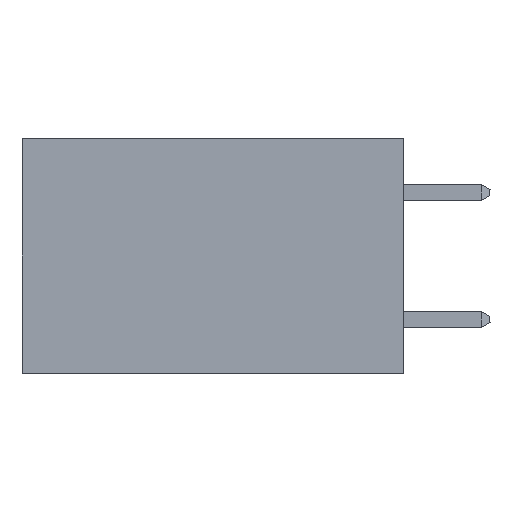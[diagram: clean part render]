
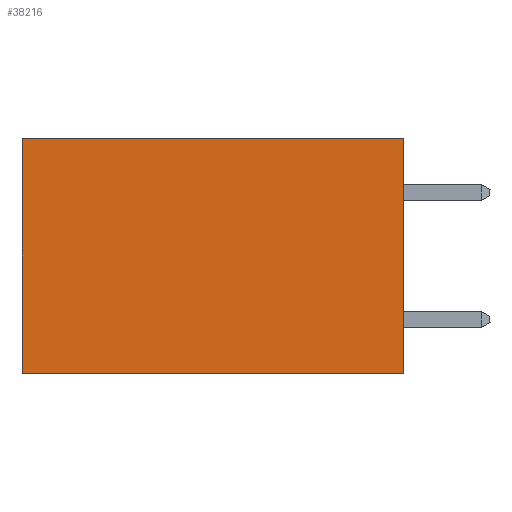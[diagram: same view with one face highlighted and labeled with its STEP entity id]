
A CAD part, left-side view. The second image highlights one B-rep face of the part: STEP entity #38216.
In plain terms, the highlighted planar face has unit normal (-1, 0, 0).
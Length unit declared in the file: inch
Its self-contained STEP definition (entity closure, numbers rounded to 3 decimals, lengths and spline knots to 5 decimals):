
#215 = CARTESIAN_POINT ( 'NONE',  ( 0.2875, 0., 0. ) ) ;
#1062 = DIRECTION ( 'NONE',  ( 0., 0., -1. ) ) ;
#1606 = EDGE_LOOP ( 'NONE', ( #6245, #32530, #17756, #23178 ) ) ;
#1956 = CARTESIAN_POINT ( 'NONE',  ( 0.2875, 0.6, -0.37 ) ) ;
#2699 = EDGE_CURVE ( 'NONE', #33863, #4896, #27996, .T. ) ;
#3627 = CARTESIAN_POINT ( 'NONE',  ( 0.2875, 0., -0.37 ) ) ;
#4805 = VECTOR ( 'NONE', #36527, 39.37008 ) ;
#4896 = VERTEX_POINT ( 'NONE', #1956 ) ;
#5256 = LINE ( 'NONE', #39238, #4805 ) ;
#6245 = ORIENTED_EDGE ( 'NONE', *, *, #2699, .T. ) ;
#9655 = VERTEX_POINT ( 'NONE', #215 ) ;
#12582 = CARTESIAN_POINT ( 'NONE',  ( 0.2875, 0., 0. ) ) ;
#15834 = PLANE ( 'NONE',  #16896 ) ;
#16367 = VECTOR ( 'NONE', #32789, 39.37008 ) ;
#16896 = AXIS2_PLACEMENT_3D ( 'NONE', #12582, #28119, #18883 ) ;
#17756 = ORIENTED_EDGE ( 'NONE', *, *, #39743, .F. ) ;
#18292 = FACE_OUTER_BOUND ( 'NONE', #1606, .T. ) ;
#18370 = VECTOR ( 'NONE', #1062, 39.37008 ) ;
#18883 = DIRECTION ( 'NONE',  ( 0., 0., -1. ) ) ;
#20125 = CARTESIAN_POINT ( 'NONE',  ( 0.2875, 0.6, 0. ) ) ;
#20802 = VECTOR ( 'NONE', #36061, 39.37008 ) ;
#23178 = ORIENTED_EDGE ( 'NONE', *, *, #31960, .T. ) ;
#27996 = LINE ( 'NONE', #20125, #16367 ) ;
#28119 = DIRECTION ( 'NONE',  ( 1., 0., 0. ) ) ;
#30313 = CARTESIAN_POINT ( 'NONE',  ( 0.2875, 0., -0.37 ) ) ;
#30358 = VERTEX_POINT ( 'NONE', #3627 ) ;
#31385 = LINE ( 'NONE', #35011, #18370 ) ;
#31960 = EDGE_CURVE ( 'NONE', #9655, #33863, #5256, .T. ) ;
#32530 = ORIENTED_EDGE ( 'NONE', *, *, #39800, .F. ) ;
#32789 = DIRECTION ( 'NONE',  ( 0., 0., -1. ) ) ;
#33784 = LINE ( 'NONE', #30313, #20802 ) ;
#33863 = VERTEX_POINT ( 'NONE', #36769 ) ;
#35011 = CARTESIAN_POINT ( 'NONE',  ( 0.2875, 0., 0. ) ) ;
#36061 = DIRECTION ( 'NONE',  ( 0., 1., 0. ) ) ;
#36527 = DIRECTION ( 'NONE',  ( 0., 1., 0. ) ) ;
#36769 = CARTESIAN_POINT ( 'NONE',  ( 0.2875, 0.6, 0. ) ) ;
#38216 = ADVANCED_FACE ( 'NONE', ( #18292 ), #15834, .F. ) ;
#39238 = CARTESIAN_POINT ( 'NONE',  ( 0.2875, 0., 0. ) ) ;
#39743 = EDGE_CURVE ( 'NONE', #9655, #30358, #31385, .T. ) ;
#39800 = EDGE_CURVE ( 'NONE', #30358, #4896, #33784, .T. ) ;
